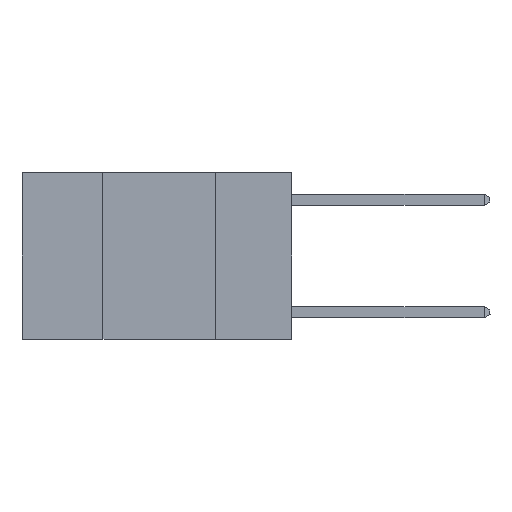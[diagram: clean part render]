
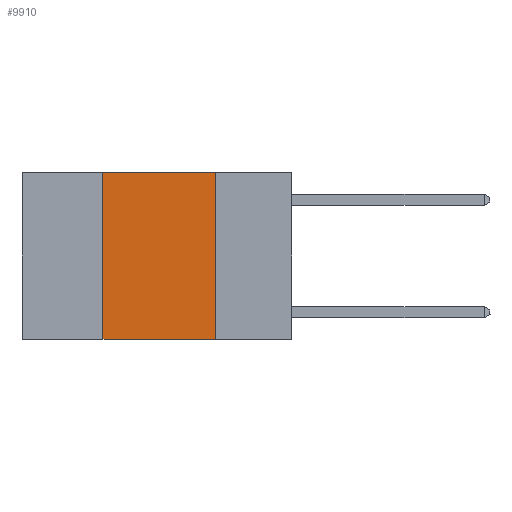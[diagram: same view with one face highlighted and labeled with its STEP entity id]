
A CAD part, left-side view. The second image highlights one B-rep face of the part: STEP entity #9910.
In plain terms, the highlighted planar face has unit normal (-1, 0, 0).
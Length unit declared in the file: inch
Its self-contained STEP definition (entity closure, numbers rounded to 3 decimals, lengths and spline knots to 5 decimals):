
#640 = EDGE_CURVE ( 'NONE', #18168, #27732, #15484, .T. ) ;
#1346 = CARTESIAN_POINT ( 'NONE',  ( 0., 0.17, 0. ) ) ;
#2195 = CARTESIAN_POINT ( 'NONE',  ( 0., 0.42, -0.37 ) ) ;
#3268 = LINE ( 'NONE', #20624, #15498 ) ;
#3308 = DIRECTION ( 'NONE',  ( 0., -1., 0. ) ) ;
#3993 = EDGE_CURVE ( 'NONE', #16890, #27732, #27871, .T. ) ;
#5330 = DIRECTION ( 'NONE',  ( 1., 0., 0. ) ) ;
#6360 = ORIENTED_EDGE ( 'NONE', *, *, #3993, .F. ) ;
#6580 = CARTESIAN_POINT ( 'NONE',  ( 0., 0.42, 0. ) ) ;
#7237 = VERTEX_POINT ( 'NONE', #21827 ) ;
#8400 = ORIENTED_EDGE ( 'NONE', *, *, #640, .T. ) ;
#9110 = FACE_OUTER_BOUND ( 'NONE', #26451, .T. ) ;
#9910 = ADVANCED_FACE ( 'NONE', ( #9110 ), #18294, .F. ) ;
#10683 = LINE ( 'NONE', #6580, #27312 ) ;
#11412 = DIRECTION ( 'NONE',  ( 0., -1., 0. ) ) ;
#11800 = CARTESIAN_POINT ( 'NONE',  ( 0., 0.6, 0. ) ) ;
#12827 = ORIENTED_EDGE ( 'NONE', *, *, #16251, .F. ) ;
#13141 = DIRECTION ( 'NONE',  ( 0., 0., 1. ) ) ;
#13859 = AXIS2_PLACEMENT_3D ( 'NONE', #11800, #5330, #20463 ) ;
#14525 = EDGE_CURVE ( 'NONE', #7237, #16890, #3268, .T. ) ;
#15484 = LINE ( 'NONE', #26562, #19847 ) ;
#15498 = VECTOR ( 'NONE', #3308, 39.37008 ) ;
#16251 = EDGE_CURVE ( 'NONE', #18168, #7237, #10683, .T. ) ;
#16308 = VECTOR ( 'NONE', #20850, 39.37008 ) ;
#16890 = VERTEX_POINT ( 'NONE', #21574 ) ;
#17866 = ORIENTED_EDGE ( 'NONE', *, *, #14525, .F. ) ;
#18168 = VERTEX_POINT ( 'NONE', #2195 ) ;
#18294 = PLANE ( 'NONE',  #13859 ) ;
#19847 = VECTOR ( 'NONE', #11412, 39.37008 ) ;
#20463 = DIRECTION ( 'NONE',  ( 0., 0., -1. ) ) ;
#20624 = CARTESIAN_POINT ( 'NONE',  ( 0., 0.6, 0. ) ) ;
#20850 = DIRECTION ( 'NONE',  ( 0., 0., -1. ) ) ;
#21574 = CARTESIAN_POINT ( 'NONE',  ( 0., 0.17, 0. ) ) ;
#21827 = CARTESIAN_POINT ( 'NONE',  ( 0., 0.42, 0. ) ) ;
#22210 = CARTESIAN_POINT ( 'NONE',  ( 0., 0.17, -0.37 ) ) ;
#26451 = EDGE_LOOP ( 'NONE', ( #6360, #17866, #12827, #8400 ) ) ;
#26562 = CARTESIAN_POINT ( 'NONE',  ( 0., 0.6, -0.37 ) ) ;
#27312 = VECTOR ( 'NONE', #13141, 39.37008 ) ;
#27732 = VERTEX_POINT ( 'NONE', #22210 ) ;
#27871 = LINE ( 'NONE', #1346, #16308 ) ;
